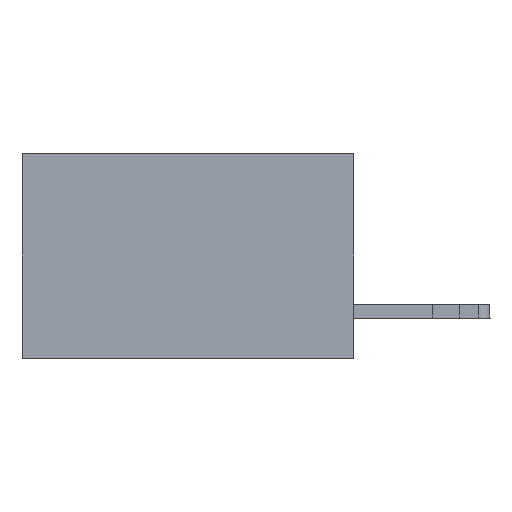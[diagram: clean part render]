
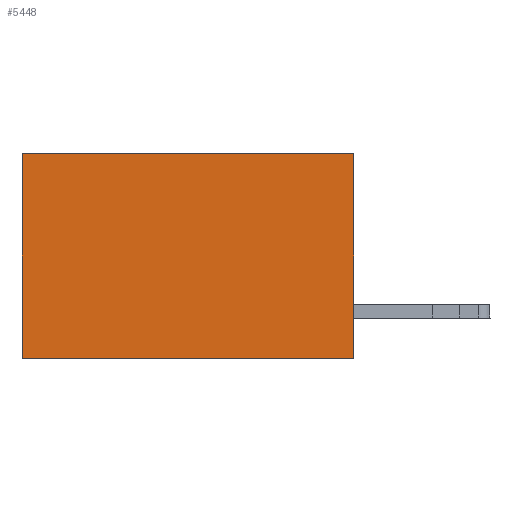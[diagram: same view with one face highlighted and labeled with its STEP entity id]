
A CAD part, left-side view. The second image highlights one B-rep face of the part: STEP entity #5448.
In plain terms, the highlighted planar face has unit normal (-1, 0, 0).
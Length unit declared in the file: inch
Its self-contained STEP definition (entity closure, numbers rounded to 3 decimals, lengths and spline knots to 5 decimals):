
#211 = CARTESIAN_POINT ( 'NONE',  ( 0.2875, 0., 0. ) ) ;
#324 = VERTEX_POINT ( 'NONE', #18920 ) ;
#384 = VECTOR ( 'NONE', #23536, 39.37008 ) ;
#791 = CARTESIAN_POINT ( 'NONE',  ( 0.2875, 0.6, -0.37 ) ) ;
#1136 = VERTEX_POINT ( 'NONE', #791 ) ;
#2306 = AXIS2_PLACEMENT_3D ( 'NONE', #211, #9504, #3799 ) ;
#2885 = VERTEX_POINT ( 'NONE', #10787 ) ;
#3569 = EDGE_CURVE ( 'NONE', #324, #1136, #15894, .T. ) ;
#3669 = DIRECTION ( 'NONE',  ( 0., 1., 0. ) ) ;
#3799 = DIRECTION ( 'NONE',  ( 0., 0., -1. ) ) ;
#4746 = CARTESIAN_POINT ( 'NONE',  ( 0.2875, 0.6, 0. ) ) ;
#5282 = VECTOR ( 'NONE', #18135, 39.37008 ) ;
#5448 = ADVANCED_FACE ( 'NONE', ( #7520 ), #22868, .F. ) ;
#5842 = VECTOR ( 'NONE', #3669, 39.37008 ) ;
#6954 = LINE ( 'NONE', #14785, #21132 ) ;
#7520 = FACE_OUTER_BOUND ( 'NONE', #24324, .T. ) ;
#7764 = CARTESIAN_POINT ( 'NONE',  ( 0.2875, 0., 0. ) ) ;
#9504 = DIRECTION ( 'NONE',  ( 1., 0., 0. ) ) ;
#10778 = ORIENTED_EDGE ( 'NONE', *, *, #19092, .F. ) ;
#10787 = CARTESIAN_POINT ( 'NONE',  ( 0.2875, 0., 0. ) ) ;
#14556 = DIRECTION ( 'NONE',  ( 0., 0., -1. ) ) ;
#14785 = CARTESIAN_POINT ( 'NONE',  ( 0.2875, 0.6, 0. ) ) ;
#15894 = LINE ( 'NONE', #16014, #384 ) ;
#16014 = CARTESIAN_POINT ( 'NONE',  ( 0.2875, 0., -0.37 ) ) ;
#17089 = LINE ( 'NONE', #7764, #5842 ) ;
#17146 = ORIENTED_EDGE ( 'NONE', *, *, #23331, .T. ) ;
#17284 = ORIENTED_EDGE ( 'NONE', *, *, #3569, .F. ) ;
#17887 = LINE ( 'NONE', #23185, #5282 ) ;
#17996 = EDGE_CURVE ( 'NONE', #22247, #1136, #6954, .T. ) ;
#18135 = DIRECTION ( 'NONE',  ( 0., 0., -1. ) ) ;
#18920 = CARTESIAN_POINT ( 'NONE',  ( 0.2875, 0., -0.37 ) ) ;
#19092 = EDGE_CURVE ( 'NONE', #2885, #324, #17887, .T. ) ;
#21132 = VECTOR ( 'NONE', #14556, 39.37008 ) ;
#22247 = VERTEX_POINT ( 'NONE', #4746 ) ;
#22695 = ORIENTED_EDGE ( 'NONE', *, *, #17996, .T. ) ;
#22868 = PLANE ( 'NONE',  #2306 ) ;
#23185 = CARTESIAN_POINT ( 'NONE',  ( 0.2875, 0., 0. ) ) ;
#23331 = EDGE_CURVE ( 'NONE', #2885, #22247, #17089, .T. ) ;
#23536 = DIRECTION ( 'NONE',  ( 0., 1., 0. ) ) ;
#24324 = EDGE_LOOP ( 'NONE', ( #22695, #17284, #10778, #17146 ) ) ;
